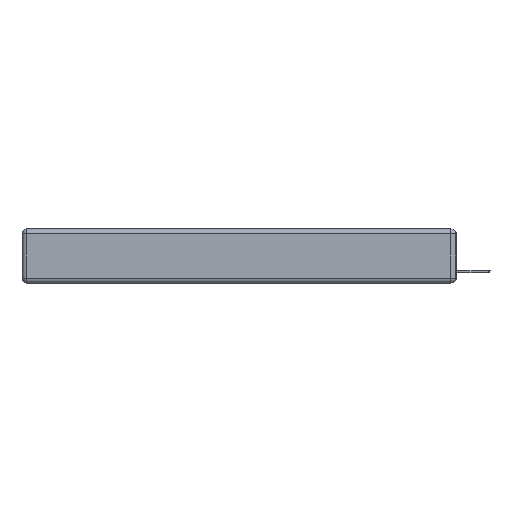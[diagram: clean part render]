
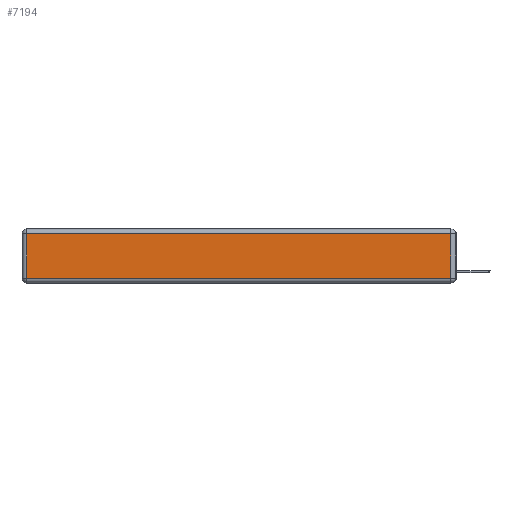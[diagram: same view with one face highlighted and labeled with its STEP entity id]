
A CAD part, left-side view. The second image highlights one B-rep face of the part: STEP entity #7194.
In plain terms, the highlighted planar face has unit normal (-1, 0, 0).
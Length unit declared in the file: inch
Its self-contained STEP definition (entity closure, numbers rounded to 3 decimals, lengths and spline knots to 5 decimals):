
#508 = VECTOR ( 'NONE', #3233, 39.37008 ) ;
#533 = EDGE_LOOP ( 'NONE', ( #6235, #7160, #4100, #1257 ) ) ;
#1010 = LINE ( 'NONE', #6827, #5920 ) ;
#1257 = ORIENTED_EDGE ( 'NONE', *, *, #4408, .T. ) ;
#1992 = LINE ( 'NONE', #10238, #508 ) ;
#2036 = CARTESIAN_POINT ( 'NONE',  ( 0., 2.72, -0.03 ) ) ;
#2275 = DIRECTION ( 'NONE',  ( 0., 0., -1. ) ) ;
#2392 = VERTEX_POINT ( 'NONE', #11009 ) ;
#3195 = CARTESIAN_POINT ( 'NONE',  ( 0., 2.72, -0.343 ) ) ;
#3220 = DIRECTION ( 'NONE',  ( 0., 0., 1. ) ) ;
#3233 = DIRECTION ( 'NONE',  ( 0., 1., 0. ) ) ;
#4100 = ORIENTED_EDGE ( 'NONE', *, *, #9793, .T. ) ;
#4408 = EDGE_CURVE ( 'NONE', #10302, #10452, #12240, .T. ) ;
#4489 = DIRECTION ( 'NONE',  ( 0., 0., 1. ) ) ;
#4557 = CARTESIAN_POINT ( 'NONE',  ( 0., 0.03, -0.03 ) ) ;
#5573 = VECTOR ( 'NONE', #4489, 39.37008 ) ;
#5920 = VECTOR ( 'NONE', #12976, 39.37008 ) ;
#6235 = ORIENTED_EDGE ( 'NONE', *, *, #11031, .T. ) ;
#6827 = CARTESIAN_POINT ( 'NONE',  ( 0., 0., -0.313 ) ) ;
#7160 = ORIENTED_EDGE ( 'NONE', *, *, #9896, .T. ) ;
#7194 = ADVANCED_FACE ( 'NONE', ( #7304 ), #11328, .T. ) ;
#7304 = FACE_OUTER_BOUND ( 'NONE', #533, .T. ) ;
#8373 = LINE ( 'NONE', #9378, #5573 ) ;
#8577 = VERTEX_POINT ( 'NONE', #4557 ) ;
#8608 = VECTOR ( 'NONE', #2275, 39.37008 ) ;
#9378 = CARTESIAN_POINT ( 'NONE',  ( 0., 0.03, -0.343 ) ) ;
#9423 = DIRECTION ( 'NONE',  ( -1., 0., 0. ) ) ;
#9793 = EDGE_CURVE ( 'NONE', #8577, #10302, #1992, .T. ) ;
#9896 = EDGE_CURVE ( 'NONE', #2392, #8577, #8373, .T. ) ;
#10238 = CARTESIAN_POINT ( 'NONE',  ( 0., 2.75, -0.03 ) ) ;
#10302 = VERTEX_POINT ( 'NONE', #2036 ) ;
#10452 = VERTEX_POINT ( 'NONE', #11394 ) ;
#11009 = CARTESIAN_POINT ( 'NONE',  ( 0., 0.03, -0.313 ) ) ;
#11031 = EDGE_CURVE ( 'NONE', #10452, #2392, #1010, .T. ) ;
#11328 = PLANE ( 'NONE',  #12501 ) ;
#11394 = CARTESIAN_POINT ( 'NONE',  ( 0., 2.72, -0.313 ) ) ;
#12240 = LINE ( 'NONE', #3195, #8608 ) ;
#12400 = CARTESIAN_POINT ( 'NONE',  ( 0., 0., -0.343 ) ) ;
#12501 = AXIS2_PLACEMENT_3D ( 'NONE', #12400, #9423, #3220 ) ;
#12976 = DIRECTION ( 'NONE',  ( 0., -1., 0. ) ) ;
